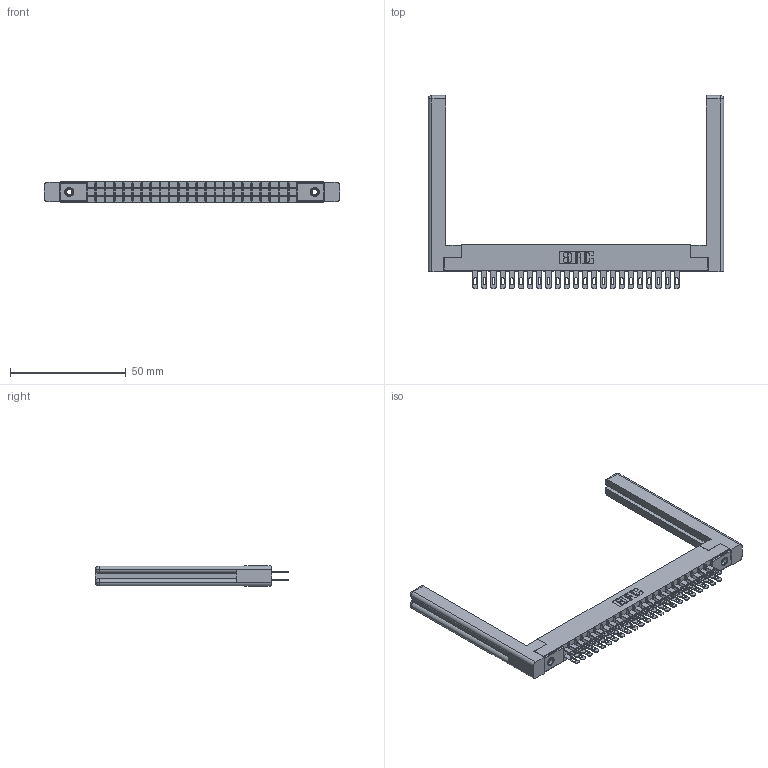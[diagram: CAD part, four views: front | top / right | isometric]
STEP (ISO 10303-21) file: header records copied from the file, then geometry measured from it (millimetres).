
FILE_DESCRIPTION (( 'STEP AP203' ), '1' );
FILE_NAME ('355-046-500-258.STEP', '2019-09-11T14:31:15', ( '' ), ( '' ), 'SwSTEP 2.0', 'SolidWorks 2016', '' );
FILE_SCHEMA (( 'CONFIG_CONTROL_DESIGN' ));
Length unit declared in the file: inch
Products named in the file (5): 307-220-058; 305 Part_.156 Dia; 345-250-001_345-250-001-102; 355-046-500-258; 305-290-001_500
Assembly tree (51 placements, depth 2):
  355-046-500-258
    305 Part_.156 Dia
    305-290-001_500  x46
    345-250-001_345-250-001-102  x2
    307-220-058  x2
Bounding box: 127.76 x 83.49 x 8.71 mm (x, y, z)
Volume: 15872.6 mm3; surface area: 21319.7 mm2
Topology: 51 solids, 51 shells, 2558 faces, 7271 edges, 4710 vertices
Faces by surface type: plane 1440, cylinder 1002, sphere 92, cone 12, torus 12
Entity records: 29871 total; most frequent: CARTESIAN_POINT 4958, ORIENTED_EDGE 4860, DIRECTION 4776, EDGE_CURVE 2430, VECTOR 1932, LINE 1932, VERTEX_POINT 1550, AXIS2_PLACEMENT_3D 1422
